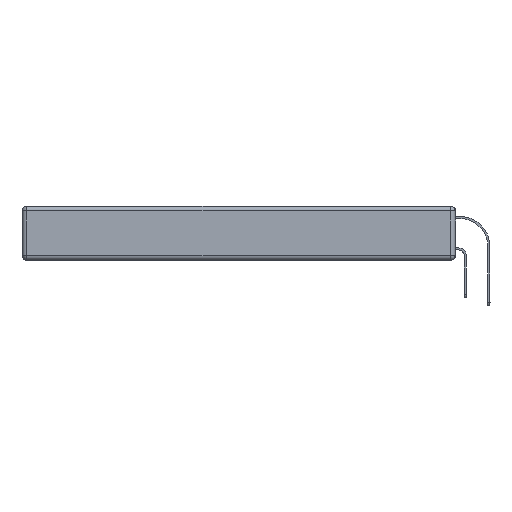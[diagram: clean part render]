
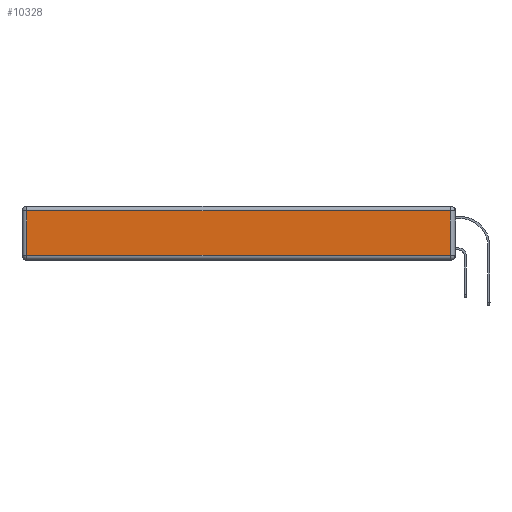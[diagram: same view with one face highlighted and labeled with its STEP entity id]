
A CAD part, left-side view. The second image highlights one B-rep face of the part: STEP entity #10328.
In plain terms, the highlighted planar face has unit normal (-1, 0, 0).
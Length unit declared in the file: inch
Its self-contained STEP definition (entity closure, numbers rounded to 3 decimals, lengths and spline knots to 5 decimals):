
#68 = EDGE_CURVE ( 'NONE', #14485, #16501, #18045, .T. ) ;
#323 = LINE ( 'NONE', #19690, #6099 ) ;
#1118 = AXIS2_PLACEMENT_3D ( 'NONE', #2040, #11182, #10198 ) ;
#1412 = ORIENTED_EDGE ( 'NONE', *, *, #8529, .T. ) ;
#1649 = VERTEX_POINT ( 'NONE', #16330 ) ;
#1891 = VERTEX_POINT ( 'NONE', #20019 ) ;
#2040 = CARTESIAN_POINT ( 'NONE',  ( 0., 0., -0.343 ) ) ;
#2373 = LINE ( 'NONE', #7470, #13812 ) ;
#2910 = EDGE_CURVE ( 'NONE', #1891, #14485, #8874, .T. ) ;
#3397 = CARTESIAN_POINT ( 'NONE',  ( 0., 0.03, -0.03 ) ) ;
#3530 = PLANE ( 'NONE',  #1118 ) ;
#4897 = VECTOR ( 'NONE', #20785, 39.37008 ) ;
#5032 = ORIENTED_EDGE ( 'NONE', *, *, #20272, .T. ) ;
#6099 = VECTOR ( 'NONE', #13470, 39.37008 ) ;
#7142 = CARTESIAN_POINT ( 'NONE',  ( 0., 2.75, -0.03 ) ) ;
#7470 = CARTESIAN_POINT ( 'NONE',  ( 0., 2.72, -0.343 ) ) ;
#8529 = EDGE_CURVE ( 'NONE', #16501, #1649, #2373, .T. ) ;
#8874 = LINE ( 'NONE', #10548, #4897 ) ;
#10198 = DIRECTION ( 'NONE',  ( 0., 0., 1. ) ) ;
#10213 = DIRECTION ( 'NONE',  ( 0., 1., 0. ) ) ;
#10328 = ADVANCED_FACE ( 'NONE', ( #18245 ), #3530, .T. ) ;
#10548 = CARTESIAN_POINT ( 'NONE',  ( 0., 0.03, -0.343 ) ) ;
#11182 = DIRECTION ( 'NONE',  ( -1., 0., 0. ) ) ;
#12123 = DIRECTION ( 'NONE',  ( 0., 0., -1. ) ) ;
#13470 = DIRECTION ( 'NONE',  ( 0., -1., 0. ) ) ;
#13812 = VECTOR ( 'NONE', #12123, 39.37008 ) ;
#14485 = VERTEX_POINT ( 'NONE', #3397 ) ;
#15021 = VECTOR ( 'NONE', #10213, 39.37008 ) ;
#15283 = ORIENTED_EDGE ( 'NONE', *, *, #68, .T. ) ;
#16263 = ORIENTED_EDGE ( 'NONE', *, *, #2910, .T. ) ;
#16330 = CARTESIAN_POINT ( 'NONE',  ( 0., 2.72, -0.313 ) ) ;
#16501 = VERTEX_POINT ( 'NONE', #20294 ) ;
#18045 = LINE ( 'NONE', #7142, #15021 ) ;
#18245 = FACE_OUTER_BOUND ( 'NONE', #19582, .T. ) ;
#19582 = EDGE_LOOP ( 'NONE', ( #5032, #16263, #15283, #1412 ) ) ;
#19690 = CARTESIAN_POINT ( 'NONE',  ( 0., 0., -0.313 ) ) ;
#20019 = CARTESIAN_POINT ( 'NONE',  ( 0., 0.03, -0.313 ) ) ;
#20272 = EDGE_CURVE ( 'NONE', #1649, #1891, #323, .T. ) ;
#20294 = CARTESIAN_POINT ( 'NONE',  ( 0., 2.72, -0.03 ) ) ;
#20785 = DIRECTION ( 'NONE',  ( 0., 0., 1. ) ) ;
